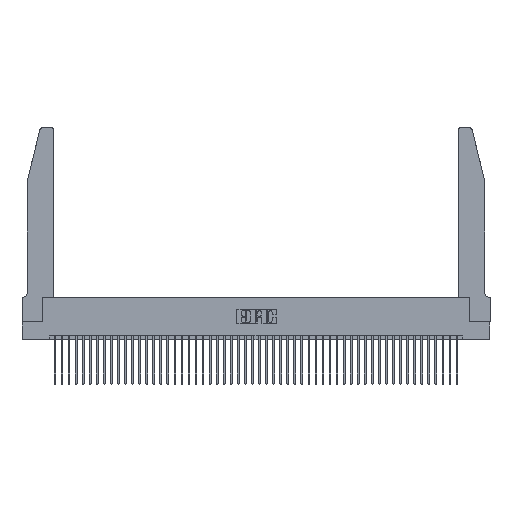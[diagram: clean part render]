
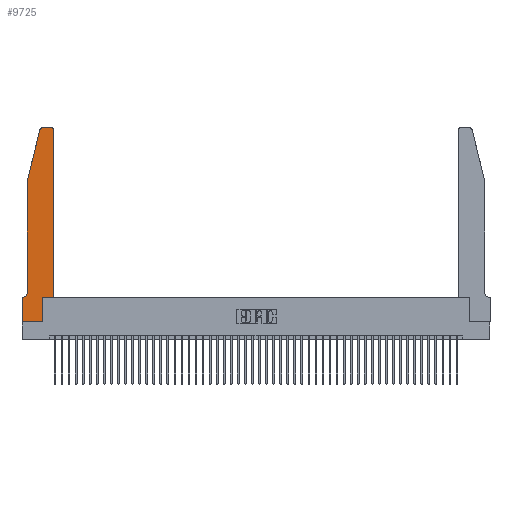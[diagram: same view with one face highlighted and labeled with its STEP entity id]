
A CAD part, top view. The second image highlights one B-rep face of the part: STEP entity #9725.
In plain terms, the highlighted planar face has unit normal (0, 0, 1).
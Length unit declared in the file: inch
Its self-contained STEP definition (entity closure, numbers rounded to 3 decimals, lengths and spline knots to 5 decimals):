
#602 = VERTEX_POINT ( 'NONE', #21245 ) ;
#792 = CARTESIAN_POINT ( 'NONE',  ( 0.2865, 0.35, 0.37 ) ) ;
#1027 = CARTESIAN_POINT ( 'NONE',  ( 0.4505, 0.35, 0.37 ) ) ;
#1147 = CIRCLE ( 'NONE', #32126, 0.03 ) ;
#1286 = VERTEX_POINT ( 'NONE', #28323 ) ;
#1440 = CARTESIAN_POINT ( 'NONE',  ( 0.4505, 0.35, 0.37 ) ) ;
#2331 = ORIENTED_EDGE ( 'NONE', *, *, #43326, .T. ) ;
#2660 = VERTEX_POINT ( 'NONE', #10167 ) ;
#3303 = EDGE_CURVE ( 'NONE', #25826, #19607, #18640, .T. ) ;
#3494 = VERTEX_POINT ( 'NONE', #35594 ) ;
#4063 = DIRECTION ( 'NONE',  ( 0., -1., 0. ) ) ;
#4507 = DIRECTION ( 'NONE',  ( 1., 0., 0. ) ) ;
#4562 = CARTESIAN_POINT ( 'NONE',  ( 0.0055, 0.35, 0.37 ) ) ;
#4921 = ORIENTED_EDGE ( 'NONE', *, *, #41647, .T. ) ;
#5664 = EDGE_LOOP ( 'NONE', ( #42954, #11223, #4921, #2331, #18199, #6042, #28904, #8626, #20038, #20641, #18904, #15856 ) ) ;
#6042 = ORIENTED_EDGE ( 'NONE', *, *, #19304, .T. ) ;
#6257 = VECTOR ( 'NONE', #34650, 39.37008 ) ;
#6698 = VECTOR ( 'NONE', #27660, 39.37008 ) ;
#8626 = ORIENTED_EDGE ( 'NONE', *, *, #28190, .T. ) ;
#8957 = DIRECTION ( 'NONE',  ( 0., -1., 0. ) ) ;
#9725 = ADVANCED_FACE ( 'NONE', ( #26362 ), #19492, .T. ) ;
#10167 = CARTESIAN_POINT ( 'NONE',  ( 0., 0., 0.37 ) ) ;
#10729 = AXIS2_PLACEMENT_3D ( 'NONE', #34172, #26929, #4507 ) ;
#10931 = VECTOR ( 'NONE', #17846, 39.37008 ) ;
#10956 = VECTOR ( 'NONE', #14217, 39.37008 ) ;
#11064 = CARTESIAN_POINT ( 'NONE',  ( 0.4205, 2.72, 0.37 ) ) ;
#11223 = ORIENTED_EDGE ( 'NONE', *, *, #24064, .T. ) ;
#12074 = LINE ( 'NONE', #31261, #30622 ) ;
#12519 = CARTESIAN_POINT ( 'NONE',  ( 0.0055, 0.42, 0.37 ) ) ;
#12604 = LINE ( 'NONE', #30841, #29986 ) ;
#13431 = DIRECTION ( 'NONE',  ( 0., 0., 1. ) ) ;
#13774 = VERTEX_POINT ( 'NONE', #29505 ) ;
#14049 = CARTESIAN_POINT ( 'NONE',  ( 0.0755, 2., 0.37 ) ) ;
#14217 = DIRECTION ( 'NONE',  ( -0.239, -0.971, 0. ) ) ;
#14530 = VERTEX_POINT ( 'NONE', #38238 ) ;
#14851 = DIRECTION ( 'NONE',  ( 1., 0., 0. ) ) ;
#15856 = ORIENTED_EDGE ( 'NONE', *, *, #44230, .T. ) ;
#16057 = EDGE_CURVE ( 'NONE', #27981, #3494, #12604, .T. ) ;
#16230 = CARTESIAN_POINT ( 'NONE',  ( 0.2865, 0.35, 0.37 ) ) ;
#16286 = DIRECTION ( 'NONE',  ( -1., 0., 0. ) ) ;
#17662 = AXIS2_PLACEMENT_3D ( 'NONE', #35520, #13431, #39221 ) ;
#17846 = DIRECTION ( 'NONE',  ( -1., 0., 0. ) ) ;
#18199 = ORIENTED_EDGE ( 'NONE', *, *, #44483, .T. ) ;
#18640 = LINE ( 'NONE', #1027, #6257 ) ;
#18904 = ORIENTED_EDGE ( 'NONE', *, *, #19658, .T. ) ;
#19304 = EDGE_CURVE ( 'NONE', #43865, #1286, #40396, .T. ) ;
#19415 = CIRCLE ( 'NONE', #21295, 0.07 ) ;
#19492 = PLANE ( 'NONE',  #10729 ) ;
#19607 = VERTEX_POINT ( 'NONE', #31047 ) ;
#19658 = EDGE_CURVE ( 'NONE', #19607, #44565, #35195, .T. ) ;
#20038 = ORIENTED_EDGE ( 'NONE', *, *, #30579, .T. ) ;
#20110 = VECTOR ( 'NONE', #8957, 39.37008 ) ;
#20237 = CARTESIAN_POINT ( 'NONE',  ( 0.0755, 2., 0.37 ) ) ;
#20641 = ORIENTED_EDGE ( 'NONE', *, *, #3303, .T. ) ;
#20845 = LINE ( 'NONE', #14049, #10956 ) ;
#21245 = CARTESIAN_POINT ( 'NONE',  ( 0.0755, 0.42, 0.37 ) ) ;
#21295 = AXIS2_PLACEMENT_3D ( 'NONE', #12519, #38324, #16286 ) ;
#22087 = CARTESIAN_POINT ( 'NONE',  ( 0.4205, 2.75, 0.37 ) ) ;
#24064 = EDGE_CURVE ( 'NONE', #3494, #13774, #26108, .T. ) ;
#24098 = VECTOR ( 'NONE', #30915, 39.37008 ) ;
#24476 = EDGE_CURVE ( 'NONE', #1286, #2660, #32146, .T. ) ;
#25826 = VERTEX_POINT ( 'NONE', #792 ) ;
#25925 = VERTEX_POINT ( 'NONE', #42275 ) ;
#26108 = CIRCLE ( 'NONE', #17662, 0.03 ) ;
#26362 = FACE_OUTER_BOUND ( 'NONE', #5664, .T. ) ;
#26487 = CARTESIAN_POINT ( 'NONE',  ( 0., 0., 0.37 ) ) ;
#26929 = DIRECTION ( 'NONE',  ( 0., 0., 1. ) ) ;
#27660 = DIRECTION ( 'NONE',  ( 0., 1., 0. ) ) ;
#27981 = VERTEX_POINT ( 'NONE', #22087 ) ;
#28190 = EDGE_CURVE ( 'NONE', #2660, #25925, #12074, .T. ) ;
#28323 = CARTESIAN_POINT ( 'NONE',  ( 0., 0.35, 0.37 ) ) ;
#28839 = CARTESIAN_POINT ( 'NONE',  ( 0.0755, 0.35, 0.37 ) ) ;
#28904 = ORIENTED_EDGE ( 'NONE', *, *, #24476, .T. ) ;
#29505 = CARTESIAN_POINT ( 'NONE',  ( 0.25487, 2.72718, 0.37 ) ) ;
#29986 = VECTOR ( 'NONE', #45595, 39.37008 ) ;
#30579 = EDGE_CURVE ( 'NONE', #25925, #25826, #35044, .T. ) ;
#30622 = VECTOR ( 'NONE', #45850, 39.37008 ) ;
#30841 = CARTESIAN_POINT ( 'NONE',  ( 0.2605, 2.75, 0.37 ) ) ;
#30915 = DIRECTION ( 'NONE',  ( 0., 1., 0. ) ) ;
#31047 = CARTESIAN_POINT ( 'NONE',  ( 0.4505, 0.35, 0.37 ) ) ;
#31261 = CARTESIAN_POINT ( 'NONE',  ( 0., 0., 0.37 ) ) ;
#32126 = AXIS2_PLACEMENT_3D ( 'NONE', #11064, #36917, #14851 ) ;
#32146 = LINE ( 'NONE', #26487, #41869 ) ;
#34172 = CARTESIAN_POINT ( 'NONE',  ( 0., 0.35, 0.37 ) ) ;
#34650 = DIRECTION ( 'NONE',  ( 1., 0., 0. ) ) ;
#35044 = LINE ( 'NONE', #16230, #24098 ) ;
#35195 = LINE ( 'NONE', #1440, #6698 ) ;
#35520 = CARTESIAN_POINT ( 'NONE',  ( 0.284, 2.72, 0.37 ) ) ;
#35594 = CARTESIAN_POINT ( 'NONE',  ( 0.284, 2.75, 0.37 ) ) ;
#36917 = DIRECTION ( 'NONE',  ( 0., 0., 1. ) ) ;
#38238 = CARTESIAN_POINT ( 'NONE',  ( 0.0755, 2., 0.37 ) ) ;
#38324 = DIRECTION ( 'NONE',  ( 0., 0., -1. ) ) ;
#39221 = DIRECTION ( 'NONE',  ( 1., 0., 0. ) ) ;
#40396 = LINE ( 'NONE', #28839, #10931 ) ;
#40831 = LINE ( 'NONE', #20237, #20110 ) ;
#41647 = EDGE_CURVE ( 'NONE', #13774, #14530, #20845, .T. ) ;
#41869 = VECTOR ( 'NONE', #4063, 39.37008 ) ;
#42275 = CARTESIAN_POINT ( 'NONE',  ( 0.2865, 0., 0.37 ) ) ;
#42337 = CARTESIAN_POINT ( 'NONE',  ( 0.4505, 2.72, 0.37 ) ) ;
#42954 = ORIENTED_EDGE ( 'NONE', *, *, #16057, .T. ) ;
#43326 = EDGE_CURVE ( 'NONE', #14530, #602, #40831, .T. ) ;
#43865 = VERTEX_POINT ( 'NONE', #4562 ) ;
#44230 = EDGE_CURVE ( 'NONE', #44565, #27981, #1147, .T. ) ;
#44483 = EDGE_CURVE ( 'NONE', #602, #43865, #19415, .T. ) ;
#44565 = VERTEX_POINT ( 'NONE', #42337 ) ;
#45595 = DIRECTION ( 'NONE',  ( -1., 0., 0. ) ) ;
#45850 = DIRECTION ( 'NONE',  ( 1., 0., 0. ) ) ;
